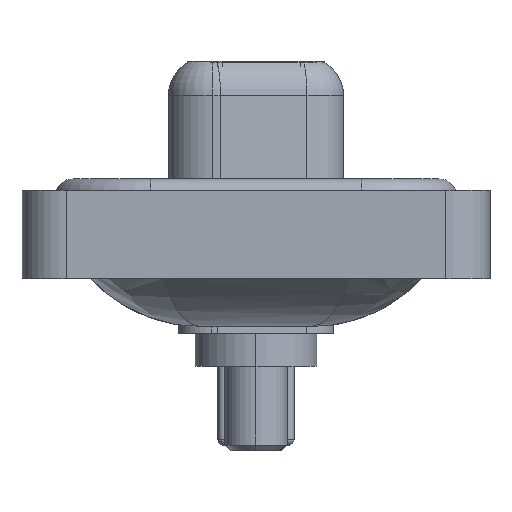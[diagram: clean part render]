
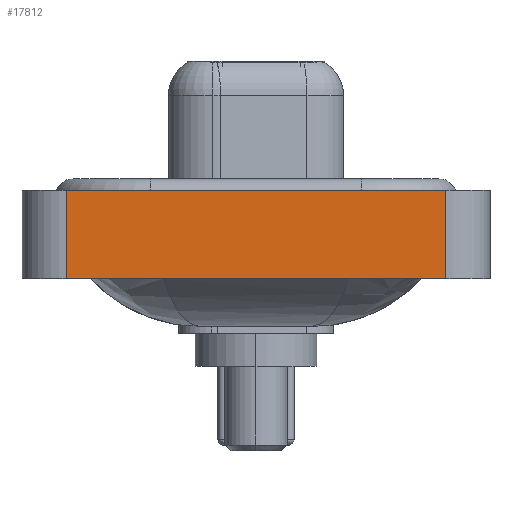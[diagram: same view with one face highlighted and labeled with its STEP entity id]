
A CAD part, left-side view. The second image highlights one B-rep face of the part: STEP entity #17812.
In plain terms, the highlighted planar face has unit normal (-1, 0, 0).
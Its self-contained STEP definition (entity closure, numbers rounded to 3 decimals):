
#927 = ORIENTED_EDGE ( 'NONE', *, *, #9662, .F. ) ;
#1548 = VERTEX_POINT ( 'NONE', #5022 ) ;
#1841 = ORIENTED_EDGE ( 'NONE', *, *, #2101, .T. ) ;
#2101 = EDGE_CURVE ( 'NONE', #1548, #8948, #3947, .T. ) ;
#2274 = CARTESIAN_POINT ( 'NONE',  ( -7.35, 8.55, -3.6 ) ) ;
#2295 = CARTESIAN_POINT ( 'NONE',  ( -7.35, -8.55, -3.6 ) ) ;
#3201 = VERTEX_POINT ( 'NONE', #22405 ) ;
#3947 = LINE ( 'NONE', #15907, #6057 ) ;
#5022 = CARTESIAN_POINT ( 'NONE',  ( -7.35, -8.55, -3.6 ) ) ;
#5202 = DIRECTION ( 'NONE',  ( -1., 0., 0. ) ) ;
#6057 = VECTOR ( 'NONE', #17746, 1000. ) ;
#6192 = VECTOR ( 'NONE', #14471, 1000. ) ;
#7316 = AXIS2_PLACEMENT_3D ( 'NONE', #16005, #5202, #9202 ) ;
#7357 = ORIENTED_EDGE ( 'NONE', *, *, #11836, .F. ) ;
#7527 = DIRECTION ( 'NONE',  ( 0., 0., 1. ) ) ;
#8920 = VERTEX_POINT ( 'NONE', #2274 ) ;
#8948 = VERTEX_POINT ( 'NONE', #20079 ) ;
#8978 = PLANE ( 'NONE',  #7316 ) ;
#9202 = DIRECTION ( 'NONE',  ( 0., 0., 1. ) ) ;
#9662 = EDGE_CURVE ( 'NONE', #3201, #8948, #15894, .T. ) ;
#11836 = EDGE_CURVE ( 'NONE', #8920, #3201, #14880, .T. ) ;
#12638 = VECTOR ( 'NONE', #7527, 1000. ) ;
#13263 = VECTOR ( 'NONE', #19877, 1000. ) ;
#14471 = DIRECTION ( 'NONE',  ( 0., -1., 0. ) ) ;
#14880 = LINE ( 'NONE', #21922, #12638 ) ;
#15894 = LINE ( 'NONE', #16555, #13263 ) ;
#15907 = CARTESIAN_POINT ( 'NONE',  ( -7.35, -8.55, -3.6 ) ) ;
#16005 = CARTESIAN_POINT ( 'NONE',  ( -7.35, -8.55, -3.6 ) ) ;
#16555 = CARTESIAN_POINT ( 'NONE',  ( -7.35, -8.55, 0.4 ) ) ;
#17746 = DIRECTION ( 'NONE',  ( 0., 0., 1. ) ) ;
#17812 = ADVANCED_FACE ( 'NONE', ( #19552 ), #8978, .T. ) ;
#18267 = LINE ( 'NONE', #2295, #6192 ) ;
#18401 = EDGE_CURVE ( 'NONE', #8920, #1548, #18267, .T. ) ;
#19149 = ORIENTED_EDGE ( 'NONE', *, *, #18401, .T. ) ;
#19552 = FACE_OUTER_BOUND ( 'NONE', #20810, .T. ) ;
#19877 = DIRECTION ( 'NONE',  ( 0., -1., 0. ) ) ;
#20079 = CARTESIAN_POINT ( 'NONE',  ( -7.35, -8.55, 0.4 ) ) ;
#20810 = EDGE_LOOP ( 'NONE', ( #1841, #927, #7357, #19149 ) ) ;
#21922 = CARTESIAN_POINT ( 'NONE',  ( -7.35, 8.55, -3.6 ) ) ;
#22405 = CARTESIAN_POINT ( 'NONE',  ( -7.35, 8.55, 0.4 ) ) ;
